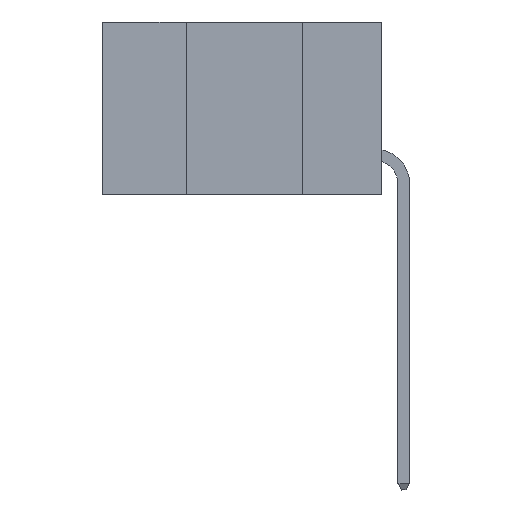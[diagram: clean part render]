
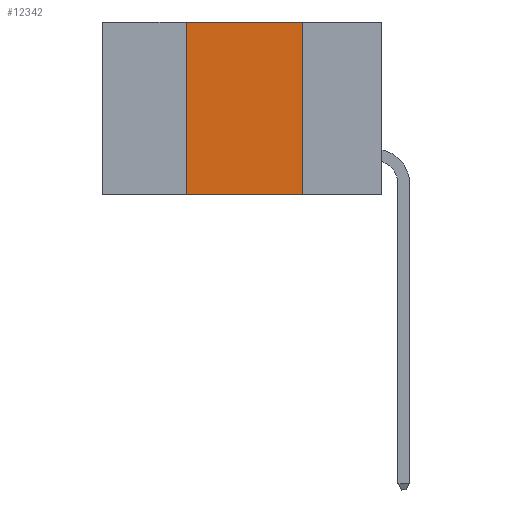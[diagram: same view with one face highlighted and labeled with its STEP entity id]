
A CAD part, left-side view. The second image highlights one B-rep face of the part: STEP entity #12342.
In plain terms, the highlighted planar face has unit normal (-1, 0, 0).
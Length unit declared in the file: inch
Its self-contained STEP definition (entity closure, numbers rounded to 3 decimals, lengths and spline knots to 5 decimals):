
#1474 = CARTESIAN_POINT ( 'NONE',  ( 0., 0.17, -0.37 ) ) ;
#2326 = VERTEX_POINT ( 'NONE', #2476 ) ;
#2457 = AXIS2_PLACEMENT_3D ( 'NONE', #13921, #12134, #24062 ) ;
#2476 = CARTESIAN_POINT ( 'NONE',  ( 0., 0.42, 0. ) ) ;
#2861 = EDGE_CURVE ( 'NONE', #17670, #12773, #12426, .T. ) ;
#3072 = CARTESIAN_POINT ( 'NONE',  ( 0., 0.42, -0.37 ) ) ;
#3206 = CARTESIAN_POINT ( 'NONE',  ( 0., 0.6, -0.37 ) ) ;
#3546 = VECTOR ( 'NONE', #11444, 39.37008 ) ;
#4199 = FACE_OUTER_BOUND ( 'NONE', #12930, .T. ) ;
#4887 = ORIENTED_EDGE ( 'NONE', *, *, #21527, .F. ) ;
#8322 = CARTESIAN_POINT ( 'NONE',  ( 0., 0.17, 0. ) ) ;
#9358 = VECTOR ( 'NONE', #26060, 39.37008 ) ;
#9661 = LINE ( 'NONE', #25972, #9358 ) ;
#9965 = VECTOR ( 'NONE', #16696, 39.37008 ) ;
#10296 = LINE ( 'NONE', #8322, #18826 ) ;
#10477 = ORIENTED_EDGE ( 'NONE', *, *, #23584, .F. ) ;
#11306 = EDGE_CURVE ( 'NONE', #24987, #12773, #10296, .T. ) ;
#11444 = DIRECTION ( 'NONE',  ( 0., -1., 0. ) ) ;
#12134 = DIRECTION ( 'NONE',  ( 1., 0., 0. ) ) ;
#12342 = ADVANCED_FACE ( 'NONE', ( #4199 ), #16041, .F. ) ;
#12426 = LINE ( 'NONE', #3206, #3546 ) ;
#12773 = VERTEX_POINT ( 'NONE', #1474 ) ;
#12930 = EDGE_LOOP ( 'NONE', ( #25873, #4887, #10477, #17235 ) ) ;
#13921 = CARTESIAN_POINT ( 'NONE',  ( 0., 0.6, 0. ) ) ;
#16041 = PLANE ( 'NONE',  #2457 ) ;
#16105 = DIRECTION ( 'NONE',  ( 0., 0., -1. ) ) ;
#16696 = DIRECTION ( 'NONE',  ( 0., 0., 1. ) ) ;
#17235 = ORIENTED_EDGE ( 'NONE', *, *, #2861, .T. ) ;
#17639 = CARTESIAN_POINT ( 'NONE',  ( 0., 0.17, 0. ) ) ;
#17670 = VERTEX_POINT ( 'NONE', #3072 ) ;
#18826 = VECTOR ( 'NONE', #16105, 39.37008 ) ;
#21527 = EDGE_CURVE ( 'NONE', #2326, #24987, #9661, .T. ) ;
#23584 = EDGE_CURVE ( 'NONE', #17670, #2326, #24523, .T. ) ;
#24062 = DIRECTION ( 'NONE',  ( 0., 0., -1. ) ) ;
#24523 = LINE ( 'NONE', #24565, #9965 ) ;
#24565 = CARTESIAN_POINT ( 'NONE',  ( 0., 0.42, 0. ) ) ;
#24987 = VERTEX_POINT ( 'NONE', #17639 ) ;
#25873 = ORIENTED_EDGE ( 'NONE', *, *, #11306, .F. ) ;
#25972 = CARTESIAN_POINT ( 'NONE',  ( 0., 0.6, 0. ) ) ;
#26060 = DIRECTION ( 'NONE',  ( 0., -1., 0. ) ) ;
